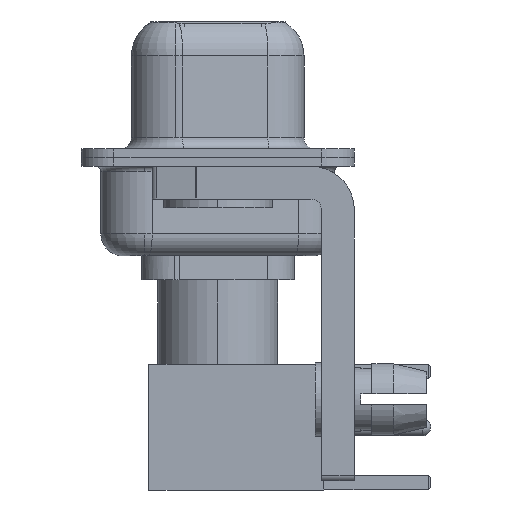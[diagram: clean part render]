
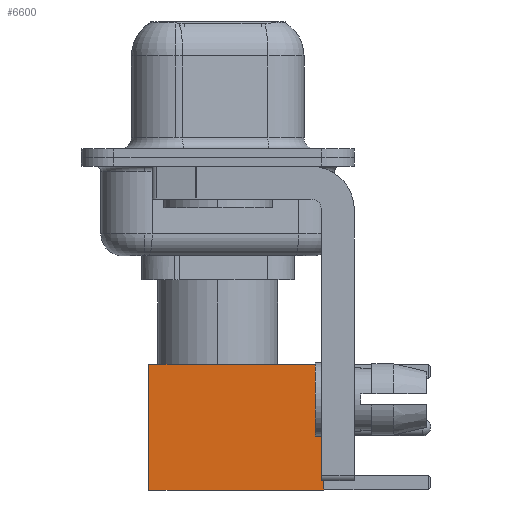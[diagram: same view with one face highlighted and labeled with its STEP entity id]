
A CAD part, left-side view. The second image highlights one B-rep face of the part: STEP entity #6600.
In plain terms, the highlighted face is planar.
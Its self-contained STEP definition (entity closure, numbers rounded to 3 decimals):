
#346 = VERTEX_POINT ( 'NONE', #10675 ) ;
#610 = ORIENTED_EDGE ( 'NONE', *, *, #6059, .T. ) ;
#662 = DIRECTION ( 'NONE',  ( 0., 1., 0. ) ) ;
#959 = DIRECTION ( 'NONE',  ( -1., 0., 0. ) ) ;
#2107 = FACE_OUTER_BOUND ( 'NONE', #8897, .T. ) ;
#2828 = VERTEX_POINT ( 'NONE', #4583 ) ;
#2887 = LINE ( 'NONE', #16197, #10788 ) ;
#3793 = CARTESIAN_POINT ( 'NONE',  ( 0., 2.875, 0. ) ) ;
#4583 = CARTESIAN_POINT ( 'NONE',  ( 2.875, 2.875, 0. ) ) ;
#4696 = EDGE_CURVE ( 'NONE', #346, #12092, #11424, .T. ) ;
#5055 = CARTESIAN_POINT ( 'NONE',  ( 2.875, 2.875, 0. ) ) ;
#6059 = EDGE_CURVE ( 'NONE', #2828, #11059, #8126, .T. ) ;
#6063 = VECTOR ( 'NONE', #959, 1000. ) ;
#6563 = VECTOR ( 'NONE', #10754, 1000. ) ;
#6600 = ADVANCED_FACE ( 'NONE', ( #2107 ), #6723, .T. ) ;
#6633 = DIRECTION ( 'NONE',  ( 0., 0., 1. ) ) ;
#6723 = PLANE ( 'NONE',  #8909 ) ;
#6955 = ORIENTED_EDGE ( 'NONE', *, *, #8785, .T. ) ;
#7842 = CARTESIAN_POINT ( 'NONE',  ( -2.875, 2.875, 0. ) ) ;
#8126 = LINE ( 'NONE', #3793, #9865 ) ;
#8785 = EDGE_CURVE ( 'NONE', #346, #2828, #2887, .T. ) ;
#8874 = DIRECTION ( 'NONE',  ( 0., 0., -1. ) ) ;
#8897 = EDGE_LOOP ( 'NONE', ( #6955, #610, #12718, #14064 ) ) ;
#8909 = AXIS2_PLACEMENT_3D ( 'NONE', #5055, #662, #6633 ) ;
#9865 = VECTOR ( 'NONE', #13726, 1000. ) ;
#10675 = CARTESIAN_POINT ( 'NONE',  ( 2.875, 2.875, 8. ) ) ;
#10754 = DIRECTION ( 'NONE',  ( 0., 0., -1. ) ) ;
#10788 = VECTOR ( 'NONE', #8874, 1000. ) ;
#11059 = VERTEX_POINT ( 'NONE', #7842 ) ;
#11424 = LINE ( 'NONE', #11624, #6063 ) ;
#11624 = CARTESIAN_POINT ( 'NONE',  ( 0., 2.875, 8. ) ) ;
#12028 = LINE ( 'NONE', #18286, #6563 ) ;
#12092 = VERTEX_POINT ( 'NONE', #17088 ) ;
#12718 = ORIENTED_EDGE ( 'NONE', *, *, #15960, .F. ) ;
#13726 = DIRECTION ( 'NONE',  ( -1., 0., 0. ) ) ;
#14064 = ORIENTED_EDGE ( 'NONE', *, *, #4696, .F. ) ;
#15960 = EDGE_CURVE ( 'NONE', #12092, #11059, #12028, .T. ) ;
#16197 = CARTESIAN_POINT ( 'NONE',  ( 2.875, 2.875, 0. ) ) ;
#17088 = CARTESIAN_POINT ( 'NONE',  ( -2.875, 2.875, 8. ) ) ;
#18286 = CARTESIAN_POINT ( 'NONE',  ( -2.875, 2.875, 0. ) ) ;
